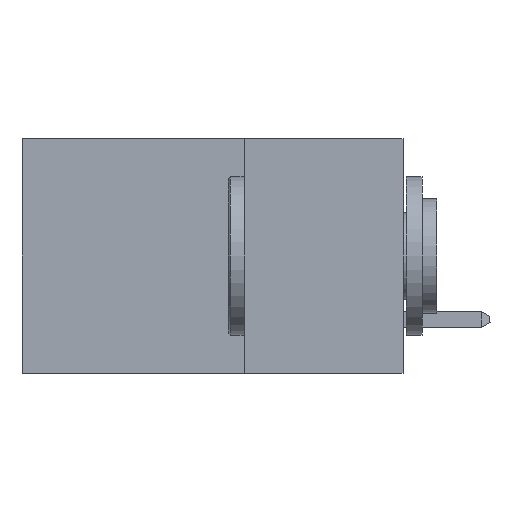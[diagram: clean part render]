
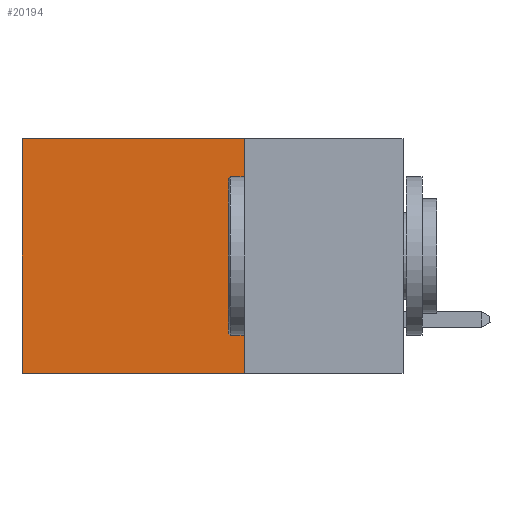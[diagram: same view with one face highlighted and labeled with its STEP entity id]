
A CAD part, left-side view. The second image highlights one B-rep face of the part: STEP entity #20194.
In plain terms, the highlighted planar face has unit normal (-1, 0, 0).
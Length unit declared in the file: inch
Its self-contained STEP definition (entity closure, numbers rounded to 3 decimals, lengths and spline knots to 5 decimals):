
#2770 = DIRECTION ( 'NONE',  ( 0., 1., 0. ) ) ;
#3193 = LINE ( 'NONE', #5690, #4135 ) ;
#3486 = PLANE ( 'NONE',  #10921 ) ;
#3789 = FACE_OUTER_BOUND ( 'NONE', #16022, .T. ) ;
#3933 = DIRECTION ( 'NONE',  ( 0., 0., -1. ) ) ;
#4103 = EDGE_CURVE ( 'NONE', #4830, #14208, #15275, .T. ) ;
#4135 = VECTOR ( 'NONE', #17911, 39.37008 ) ;
#4178 = CARTESIAN_POINT ( 'NONE',  ( 0.2875, 0.25, 0. ) ) ;
#4292 = ORIENTED_EDGE ( 'NONE', *, *, #4103, .F. ) ;
#4526 = ORIENTED_EDGE ( 'NONE', *, *, #18204, .T. ) ;
#4830 = VERTEX_POINT ( 'NONE', #6812 ) ;
#5167 = LINE ( 'NONE', #11538, #6458 ) ;
#5690 = CARTESIAN_POINT ( 'NONE',  ( 0.2875, 0.25, 0. ) ) ;
#5825 = VERTEX_POINT ( 'NONE', #10743 ) ;
#6146 = VECTOR ( 'NONE', #2770, 39.37008 ) ;
#6279 = EDGE_CURVE ( 'NONE', #24607, #4830, #3193, .T. ) ;
#6458 = VECTOR ( 'NONE', #19178, 39.37008 ) ;
#6812 = CARTESIAN_POINT ( 'NONE',  ( 0.2875, 0.25, -0.37 ) ) ;
#9251 = VECTOR ( 'NONE', #24965, 39.37008 ) ;
#10743 = CARTESIAN_POINT ( 'NONE',  ( 0.2875, 0.6, 0. ) ) ;
#10921 = AXIS2_PLACEMENT_3D ( 'NONE', #11456, #25549, #3933 ) ;
#11456 = CARTESIAN_POINT ( 'NONE',  ( 0.2875, 0.25, 0. ) ) ;
#11538 = CARTESIAN_POINT ( 'NONE',  ( 0.2875, 0.6, 0. ) ) ;
#13679 = EDGE_CURVE ( 'NONE', #5825, #14208, #5167, .T. ) ;
#14208 = VERTEX_POINT ( 'NONE', #21187 ) ;
#14610 = LINE ( 'NONE', #20988, #9251 ) ;
#15046 = CARTESIAN_POINT ( 'NONE',  ( 0.2875, 0.25, -0.37 ) ) ;
#15275 = LINE ( 'NONE', #15046, #6146 ) ;
#16022 = EDGE_LOOP ( 'NONE', ( #25622, #4292, #19450, #4526 ) ) ;
#17911 = DIRECTION ( 'NONE',  ( 0., 0., -1. ) ) ;
#18204 = EDGE_CURVE ( 'NONE', #24607, #5825, #14610, .T. ) ;
#19178 = DIRECTION ( 'NONE',  ( 0., 0., -1. ) ) ;
#19450 = ORIENTED_EDGE ( 'NONE', *, *, #6279, .F. ) ;
#20194 = ADVANCED_FACE ( 'NONE', ( #3789 ), #3486, .F. ) ;
#20988 = CARTESIAN_POINT ( 'NONE',  ( 0.2875, 0.25, 0. ) ) ;
#21187 = CARTESIAN_POINT ( 'NONE',  ( 0.2875, 0.6, -0.37 ) ) ;
#24607 = VERTEX_POINT ( 'NONE', #4178 ) ;
#24965 = DIRECTION ( 'NONE',  ( 0., 1., 0. ) ) ;
#25549 = DIRECTION ( 'NONE',  ( 1., 0., 0. ) ) ;
#25622 = ORIENTED_EDGE ( 'NONE', *, *, #13679, .T. ) ;
